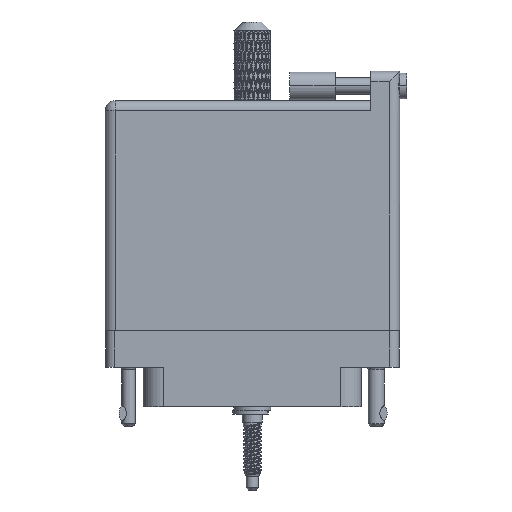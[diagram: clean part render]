
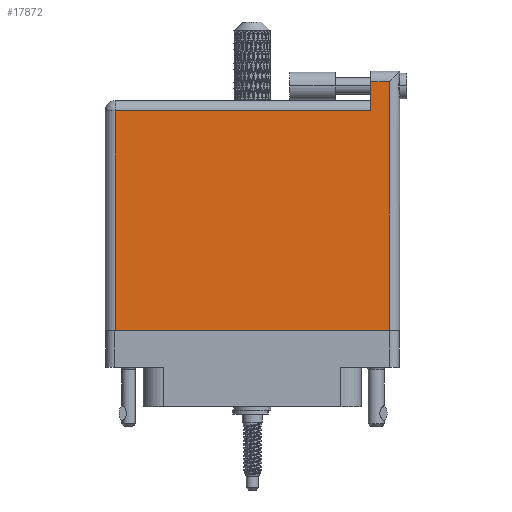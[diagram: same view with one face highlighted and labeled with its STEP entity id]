
A CAD part, front view. The second image highlights one B-rep face of the part: STEP entity #17872.
In plain terms, the highlighted face is planar.
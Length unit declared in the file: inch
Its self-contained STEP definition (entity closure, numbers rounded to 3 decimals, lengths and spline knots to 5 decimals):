
#2569 = EDGE_CURVE ( 'NONE', #76275, #47495, #91144, .T. ) ;
#5837 = ORIENTED_EDGE ( 'NONE', *, *, #53010, .T. ) ;
#5846 = LINE ( 'NONE', #27254, #48719 ) ;
#9210 = DIRECTION ( 'NONE',  ( -1., 0., 0. ) ) ;
#10123 = DIRECTION ( 'NONE',  ( -1., 0., 0. ) ) ;
#10223 = DIRECTION ( 'NONE',  ( -1., 0., 0. ) ) ;
#11116 = ORIENTED_EDGE ( 'NONE', *, *, #2569, .T. ) ;
#13899 = EDGE_CURVE ( 'NONE', #52297, #101058, #62079, .T. ) ;
#14261 = EDGE_CURVE ( 'NONE', #71956, #92398, #44718, .T. ) ;
#15220 = VECTOR ( 'NONE', #10123, 39.37008 ) ;
#17872 = ADVANCED_FACE ( 'NONE', ( #57461 ), #78766, .F. ) ;
#17979 = LINE ( 'NONE', #77444, #87706 ) ;
#24775 = ORIENTED_EDGE ( 'NONE', *, *, #68539, .T. ) ;
#25194 = CARTESIAN_POINT ( 'NONE',  ( 0.807, 1.596, 0.4495 ) ) ;
#27254 = CARTESIAN_POINT ( 'NONE',  ( 0.807, 1.666, 0.4495 ) ) ;
#32195 = VECTOR ( 'NONE', #67230, 39.37008 ) ;
#32652 = CARTESIAN_POINT ( 'NONE',  ( 0.807, 1.396, 0.4495 ) ) ;
#44718 = LINE ( 'NONE', #79410, #104922 ) ;
#47495 = VERTEX_POINT ( 'NONE', #69666 ) ;
#48719 = VECTOR ( 'NONE', #61624, 39.37008 ) ;
#50384 = CARTESIAN_POINT ( 'NONE',  ( -1.004, -0.1, 0.4495 ) ) ;
#51381 = DIRECTION ( 'NONE',  ( 0., -1., 0. ) ) ;
#52274 = CARTESIAN_POINT ( 'NONE',  ( 0.934, 1.596, 0.4495 ) ) ;
#52297 = VERTEX_POINT ( 'NONE', #32652 ) ;
#53010 = EDGE_CURVE ( 'NONE', #101058, #76275, #87593, .T. ) ;
#53093 = CARTESIAN_POINT ( 'NONE',  ( -0.934, 1.396, 0.4495 ) ) ;
#57461 = FACE_OUTER_BOUND ( 'NONE', #105816, .T. ) ;
#60453 = CARTESIAN_POINT ( 'NONE',  ( -1.004, 1.466, 0.4495 ) ) ;
#61624 = DIRECTION ( 'NONE',  ( 0., -1., 0. ) ) ;
#62079 = LINE ( 'NONE', #95801, #15220 ) ;
#66084 = VECTOR ( 'NONE', #51381, 39.37008 ) ;
#67230 = DIRECTION ( 'NONE',  ( 1., 0., 0. ) ) ;
#68539 = EDGE_CURVE ( 'NONE', #92398, #52297, #5846, .T. ) ;
#69093 = DIRECTION ( 'NONE',  ( 0., 0., -1. ) ) ;
#69666 = CARTESIAN_POINT ( 'NONE',  ( 0.934, -0.1, 0.4495 ) ) ;
#71710 = ORIENTED_EDGE ( 'NONE', *, *, #14261, .T. ) ;
#71956 = VERTEX_POINT ( 'NONE', #52274 ) ;
#76275 = VERTEX_POINT ( 'NONE', #87866 ) ;
#76746 = DIRECTION ( 'NONE',  ( 0., 1., 0. ) ) ;
#77403 = AXIS2_PLACEMENT_3D ( 'NONE', #60453, #69093, #9210 ) ;
#77444 = CARTESIAN_POINT ( 'NONE',  ( 0.934, 1.666, 0.4495 ) ) ;
#77667 = ORIENTED_EDGE ( 'NONE', *, *, #13899, .T. ) ;
#78766 = PLANE ( 'NONE',  #77403 ) ;
#79410 = CARTESIAN_POINT ( 'NONE',  ( -1.004, 1.596, 0.4495 ) ) ;
#87593 = LINE ( 'NONE', #102658, #66084 ) ;
#87706 = VECTOR ( 'NONE', #76746, 39.37008 ) ;
#87866 = CARTESIAN_POINT ( 'NONE',  ( -0.934, -0.1, 0.4495 ) ) ;
#91144 = LINE ( 'NONE', #50384, #32195 ) ;
#92398 = VERTEX_POINT ( 'NONE', #25194 ) ;
#94267 = EDGE_CURVE ( 'NONE', #47495, #71956, #17979, .T. ) ;
#95801 = CARTESIAN_POINT ( 'NONE',  ( -1.004, 1.396, 0.4495 ) ) ;
#101058 = VERTEX_POINT ( 'NONE', #53093 ) ;
#102658 = CARTESIAN_POINT ( 'NONE',  ( -0.934, -0.1, 0.4495 ) ) ;
#104922 = VECTOR ( 'NONE', #10223, 39.37008 ) ;
#105816 = EDGE_LOOP ( 'NONE', ( #11116, #108517, #71710, #24775, #77667, #5837 ) ) ;
#108517 = ORIENTED_EDGE ( 'NONE', *, *, #94267, .T. ) ;
